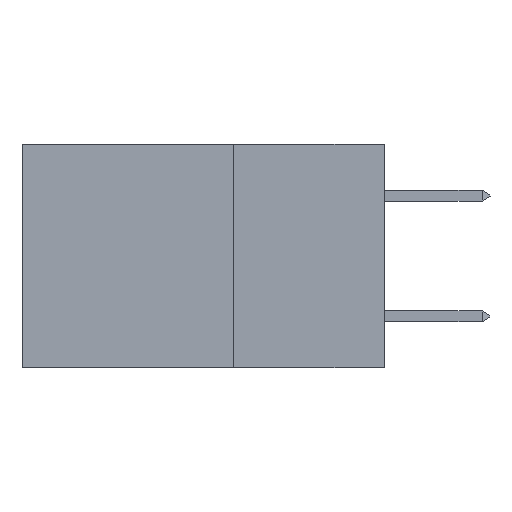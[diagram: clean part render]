
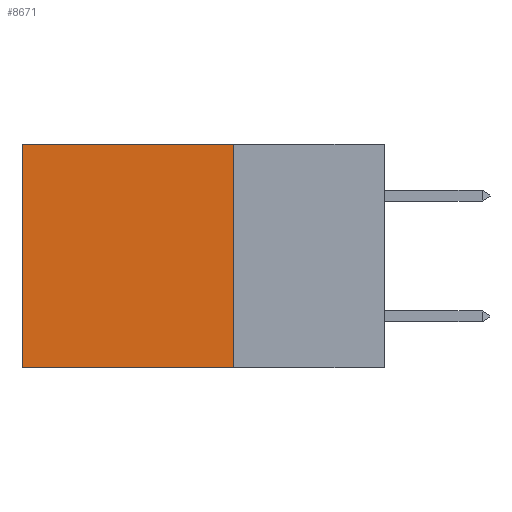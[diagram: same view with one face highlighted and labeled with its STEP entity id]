
A CAD part, left-side view. The second image highlights one B-rep face of the part: STEP entity #8671.
In plain terms, the highlighted planar face has unit normal (-1, 0, 0).
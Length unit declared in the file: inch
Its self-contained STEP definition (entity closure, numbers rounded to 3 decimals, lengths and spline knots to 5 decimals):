
#178 = LINE ( 'NONE', #8919, #8780 ) ;
#303 = VERTEX_POINT ( 'NONE', #701 ) ;
#335 = ORIENTED_EDGE ( 'NONE', *, *, #9264, .T. ) ;
#701 = CARTESIAN_POINT ( 'NONE',  ( 0.2875, 0.6, 0. ) ) ;
#1518 = CARTESIAN_POINT ( 'NONE',  ( 0.2875, 0.25, 0. ) ) ;
#2998 = VECTOR ( 'NONE', #6872, 39.37008 ) ;
#3025 = CARTESIAN_POINT ( 'NONE',  ( 0.2875, 0.25, 0. ) ) ;
#3208 = EDGE_LOOP ( 'NONE', ( #335, #7884, #5609, #7539 ) ) ;
#3362 = VERTEX_POINT ( 'NONE', #6021 ) ;
#3520 = DIRECTION ( 'NONE',  ( 0., 0., -1. ) ) ;
#3891 = AXIS2_PLACEMENT_3D ( 'NONE', #1518, #7233, #3520 ) ;
#4240 = DIRECTION ( 'NONE',  ( 0., 1., 0. ) ) ;
#4299 = PLANE ( 'NONE',  #3891 ) ;
#4316 = CARTESIAN_POINT ( 'NONE',  ( 0.2875, 0.25, 0. ) ) ;
#5536 = EDGE_CURVE ( 'NONE', #12364, #10384, #9896, .T. ) ;
#5609 = ORIENTED_EDGE ( 'NONE', *, *, #5536, .F. ) ;
#5689 = EDGE_CURVE ( 'NONE', #12364, #303, #11053, .T. ) ;
#6021 = CARTESIAN_POINT ( 'NONE',  ( 0.2875, 0.6, -0.37 ) ) ;
#6709 = CARTESIAN_POINT ( 'NONE',  ( 0.2875, 0.25, -0.37 ) ) ;
#6872 = DIRECTION ( 'NONE',  ( 0., 0., -1. ) ) ;
#7222 = EDGE_CURVE ( 'NONE', #10384, #3362, #178, .T. ) ;
#7233 = DIRECTION ( 'NONE',  ( 1., 0., 0. ) ) ;
#7363 = FACE_OUTER_BOUND ( 'NONE', #3208, .T. ) ;
#7539 = ORIENTED_EDGE ( 'NONE', *, *, #5689, .T. ) ;
#7760 = DIRECTION ( 'NONE',  ( 0., 1., 0. ) ) ;
#7884 = ORIENTED_EDGE ( 'NONE', *, *, #7222, .F. ) ;
#8309 = VECTOR ( 'NONE', #11596, 39.37008 ) ;
#8581 = CARTESIAN_POINT ( 'NONE',  ( 0.2875, 0.6, 0. ) ) ;
#8671 = ADVANCED_FACE ( 'NONE', ( #7363 ), #4299, .F. ) ;
#8780 = VECTOR ( 'NONE', #7760, 39.37008 ) ;
#8919 = CARTESIAN_POINT ( 'NONE',  ( 0.2875, 0.25, -0.37 ) ) ;
#9264 = EDGE_CURVE ( 'NONE', #303, #3362, #9537, .T. ) ;
#9537 = LINE ( 'NONE', #8581, #8309 ) ;
#9896 = LINE ( 'NONE', #3025, #2998 ) ;
#10087 = CARTESIAN_POINT ( 'NONE',  ( 0.2875, 0.25, 0. ) ) ;
#10384 = VERTEX_POINT ( 'NONE', #6709 ) ;
#11053 = LINE ( 'NONE', #10087, #11628 ) ;
#11596 = DIRECTION ( 'NONE',  ( 0., 0., -1. ) ) ;
#11628 = VECTOR ( 'NONE', #4240, 39.37008 ) ;
#12364 = VERTEX_POINT ( 'NONE', #4316 ) ;
